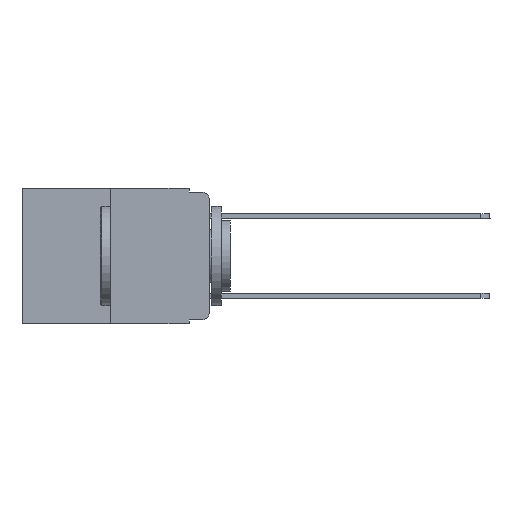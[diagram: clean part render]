
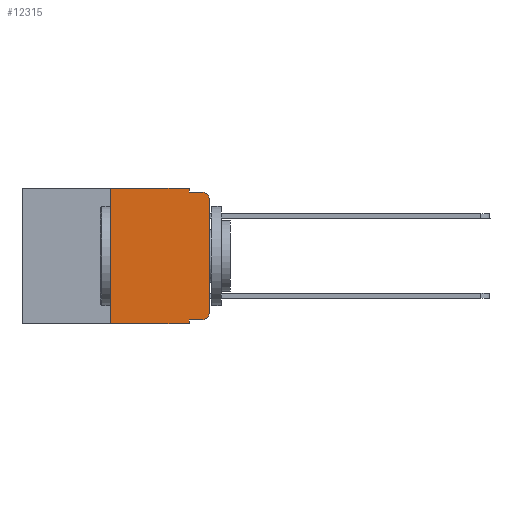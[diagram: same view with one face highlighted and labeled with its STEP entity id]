
A CAD part, left-side view. The second image highlights one B-rep face of the part: STEP entity #12315.
In plain terms, the highlighted planar face has unit normal (-1, 0, 0).
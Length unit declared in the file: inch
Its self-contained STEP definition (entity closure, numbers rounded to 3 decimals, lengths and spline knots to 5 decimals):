
#47 = EDGE_CURVE ( 'NONE', #15195, #15107, #53, .T. ) ;
#53 = LINE ( 'NONE', #15463, #4759 ) ;
#271 = VECTOR ( 'NONE', #5911, 39.37008 ) ;
#323 = CARTESIAN_POINT ( 'NONE',  ( 0., 0.25, 0. ) ) ;
#456 = DIRECTION ( 'NONE',  ( 0., 0., 1. ) ) ;
#688 = LINE ( 'NONE', #23744, #24105 ) ;
#1030 = DIRECTION ( 'NONE',  ( 0., -1., 0. ) ) ;
#1748 = CARTESIAN_POINT ( 'NONE',  ( 0., 0.051, -0.01 ) ) ;
#1849 = ORIENTED_EDGE ( 'NONE', *, *, #12424, .T. ) ;
#2281 = DIRECTION ( 'NONE',  ( 0., 0., -1. ) ) ;
#2408 = LINE ( 'NONE', #24127, #5605 ) ;
#3001 = CARTESIAN_POINT ( 'NONE',  ( 0., 0.051, -0.333 ) ) ;
#3137 = DIRECTION ( 'NONE',  ( -1., 0., 0. ) ) ;
#3281 = CARTESIAN_POINT ( 'NONE',  ( 0., 0.051, -0.01 ) ) ;
#3723 = ORIENTED_EDGE ( 'NONE', *, *, #15292, .F. ) ;
#4288 = VERTEX_POINT ( 'NONE', #23311 ) ;
#4640 = CARTESIAN_POINT ( 'NONE',  ( 0., 0.25, 0. ) ) ;
#4759 = VECTOR ( 'NONE', #25358, 39.37008 ) ;
#4982 = CARTESIAN_POINT ( 'NONE',  ( 0., 0.02, -0.03 ) ) ;
#5383 = EDGE_CURVE ( 'NONE', #4288, #5551, #2408, .T. ) ;
#5519 = VERTEX_POINT ( 'NONE', #14863 ) ;
#5551 = VERTEX_POINT ( 'NONE', #18586 ) ;
#5605 = VECTOR ( 'NONE', #13968, 39.37008 ) ;
#5620 = ORIENTED_EDGE ( 'NONE', *, *, #47, .T. ) ;
#5911 = DIRECTION ( 'NONE',  ( 0., -1., 0. ) ) ;
#6087 = CIRCLE ( 'NONE', #21711, 0.02 ) ;
#6475 = PLANE ( 'NONE',  #13486 ) ;
#6581 = CARTESIAN_POINT ( 'NONE',  ( 0., 0.473, 0. ) ) ;
#7130 = ORIENTED_EDGE ( 'NONE', *, *, #13245, .F. ) ;
#8679 = EDGE_CURVE ( 'NONE', #4288, #23209, #10578, .T. ) ;
#9694 = AXIS2_PLACEMENT_3D ( 'NONE', #4982, #16675, #12811 ) ;
#10260 = EDGE_CURVE ( 'NONE', #18667, #5519, #25357, .T. ) ;
#10578 = LINE ( 'NONE', #323, #16242 ) ;
#11340 = DIRECTION ( 'NONE',  ( 0., 0., -1. ) ) ;
#12315 = ADVANCED_FACE ( 'NONE', ( #24098 ), #6475, .F. ) ;
#12424 = EDGE_CURVE ( 'NONE', #5519, #15195, #6087, .T. ) ;
#12764 = EDGE_CURVE ( 'NONE', #23209, #24973, #17877, .T. ) ;
#12811 = DIRECTION ( 'NONE',  ( 0., 0., -1. ) ) ;
#13177 = LINE ( 'NONE', #1748, #15598 ) ;
#13245 = EDGE_CURVE ( 'NONE', #18306, #20632, #13177, .T. ) ;
#13486 = AXIS2_PLACEMENT_3D ( 'NONE', #14324, #24843, #20889 ) ;
#13601 = CARTESIAN_POINT ( 'NONE',  ( 0., 0.051, 0. ) ) ;
#13968 = DIRECTION ( 'NONE',  ( 0., -1., 0. ) ) ;
#14324 = CARTESIAN_POINT ( 'NONE',  ( 0., 0.473, 0. ) ) ;
#14340 = VECTOR ( 'NONE', #14421, 39.37008 ) ;
#14421 = DIRECTION ( 'NONE',  ( 0., -1., 0. ) ) ;
#14776 = ORIENTED_EDGE ( 'NONE', *, *, #8679, .F. ) ;
#14863 = CARTESIAN_POINT ( 'NONE',  ( 0., 0.02, -0.333 ) ) ;
#14935 = EDGE_CURVE ( 'NONE', #15107, #20632, #23686, .T. ) ;
#15107 = VERTEX_POINT ( 'NONE', #21427 ) ;
#15195 = VERTEX_POINT ( 'NONE', #15509 ) ;
#15292 = EDGE_CURVE ( 'NONE', #18667, #5551, #688, .T. ) ;
#15463 = CARTESIAN_POINT ( 'NONE',  ( 0., 0., 0. ) ) ;
#15509 = CARTESIAN_POINT ( 'NONE',  ( 0., 0., -0.313 ) ) ;
#15548 = ORIENTED_EDGE ( 'NONE', *, *, #5383, .T. ) ;
#15598 = VECTOR ( 'NONE', #1030, 39.37008 ) ;
#15949 = VECTOR ( 'NONE', #2281, 39.37008 ) ;
#16242 = VECTOR ( 'NONE', #456, 39.37008 ) ;
#16542 = EDGE_LOOP ( 'NONE', ( #5620, #18907, #7130, #22972, #19216, #14776, #15548, #3723, #24646, #1849 ) ) ;
#16675 = DIRECTION ( 'NONE',  ( -1., 0., 0. ) ) ;
#17877 = LINE ( 'NONE', #6581, #14340 ) ;
#18306 = VERTEX_POINT ( 'NONE', #3281 ) ;
#18586 = CARTESIAN_POINT ( 'NONE',  ( 0., 0.051, -0.343 ) ) ;
#18667 = VERTEX_POINT ( 'NONE', #3001 ) ;
#18907 = ORIENTED_EDGE ( 'NONE', *, *, #14935, .T. ) ;
#19216 = ORIENTED_EDGE ( 'NONE', *, *, #12764, .F. ) ;
#20066 = CARTESIAN_POINT ( 'NONE',  ( 0., 0.02, -0.01 ) ) ;
#20632 = VERTEX_POINT ( 'NONE', #20066 ) ;
#20889 = DIRECTION ( 'NONE',  ( 0., 0., -1. ) ) ;
#21427 = CARTESIAN_POINT ( 'NONE',  ( 0., 0., -0.03 ) ) ;
#21497 = CARTESIAN_POINT ( 'NONE',  ( 0., 0.051, -0.333 ) ) ;
#21711 = AXIS2_PLACEMENT_3D ( 'NONE', #22686, #3137, #11340 ) ;
#21839 = CARTESIAN_POINT ( 'NONE',  ( 0., 0.051, 0. ) ) ;
#22686 = CARTESIAN_POINT ( 'NONE',  ( 0., 0.02, -0.313 ) ) ;
#22972 = ORIENTED_EDGE ( 'NONE', *, *, #24920, .F. ) ;
#23209 = VERTEX_POINT ( 'NONE', #4640 ) ;
#23311 = CARTESIAN_POINT ( 'NONE',  ( 0., 0.25, -0.343 ) ) ;
#23686 = CIRCLE ( 'NONE', #9694, 0.02 ) ;
#23744 = CARTESIAN_POINT ( 'NONE',  ( 0., 0.051, 0. ) ) ;
#24005 = LINE ( 'NONE', #21839, #15949 ) ;
#24098 = FACE_OUTER_BOUND ( 'NONE', #16542, .T. ) ;
#24105 = VECTOR ( 'NONE', #24221, 39.37008 ) ;
#24127 = CARTESIAN_POINT ( 'NONE',  ( 0., 0.473, -0.343 ) ) ;
#24221 = DIRECTION ( 'NONE',  ( 0., 0., -1. ) ) ;
#24646 = ORIENTED_EDGE ( 'NONE', *, *, #10260, .T. ) ;
#24843 = DIRECTION ( 'NONE',  ( 1., 0., 0. ) ) ;
#24920 = EDGE_CURVE ( 'NONE', #24973, #18306, #24005, .T. ) ;
#24973 = VERTEX_POINT ( 'NONE', #13601 ) ;
#25357 = LINE ( 'NONE', #21497, #271 ) ;
#25358 = DIRECTION ( 'NONE',  ( 0., 0., 1. ) ) ;
